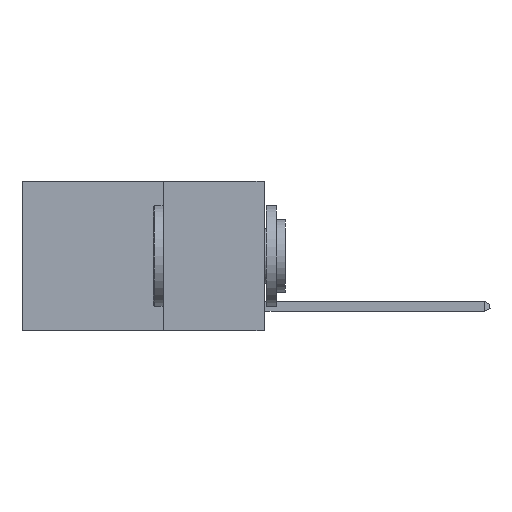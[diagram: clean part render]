
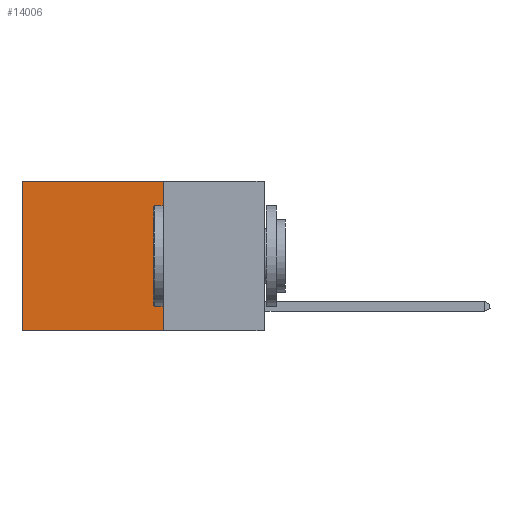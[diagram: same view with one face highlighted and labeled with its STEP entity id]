
A CAD part, left-side view. The second image highlights one B-rep face of the part: STEP entity #14006.
In plain terms, the highlighted planar face has unit normal (-1, 0, 0).
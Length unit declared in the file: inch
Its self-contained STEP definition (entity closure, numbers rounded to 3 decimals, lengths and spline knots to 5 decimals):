
#218 = DIRECTION ( 'NONE',  ( 0., 1., 0. ) ) ;
#774 = EDGE_CURVE ( 'NONE', #12785, #7428, #1896, .T. ) ;
#1178 = CARTESIAN_POINT ( 'NONE',  ( 0.2625, 0.25, 0. ) ) ;
#1499 = ORIENTED_EDGE ( 'NONE', *, *, #6304, .T. ) ;
#1896 = LINE ( 'NONE', #18213, #20270 ) ;
#2748 = EDGE_CURVE ( 'NONE', #5955, #7428, #11706, .T. ) ;
#3191 = PLANE ( 'NONE',  #17460 ) ;
#4919 = DIRECTION ( 'NONE',  ( 1., 0., 0. ) ) ;
#5217 = CARTESIAN_POINT ( 'NONE',  ( 0.2625, 0.6, 0. ) ) ;
#5929 = DIRECTION ( 'NONE',  ( 0., 0., -1. ) ) ;
#5955 = VERTEX_POINT ( 'NONE', #5217 ) ;
#6304 = EDGE_CURVE ( 'NONE', #12849, #5955, #6588, .T. ) ;
#6588 = LINE ( 'NONE', #6692, #6693 ) ;
#6692 = CARTESIAN_POINT ( 'NONE',  ( 0.2625, 0.25, 0. ) ) ;
#6693 = VECTOR ( 'NONE', #218, 39.37008 ) ;
#7428 = VERTEX_POINT ( 'NONE', #13947 ) ;
#7990 = ORIENTED_EDGE ( 'NONE', *, *, #17833, .F. ) ;
#8129 = DIRECTION ( 'NONE',  ( 0., 0., -1. ) ) ;
#10306 = CARTESIAN_POINT ( 'NONE',  ( 0.2625, 0.25, 0. ) ) ;
#11030 = EDGE_LOOP ( 'NONE', ( #17191, #18060, #7990, #1499 ) ) ;
#11706 = LINE ( 'NONE', #18285, #13507 ) ;
#12785 = VERTEX_POINT ( 'NONE', #21215 ) ;
#12849 = VERTEX_POINT ( 'NONE', #10306 ) ;
#13134 = FACE_OUTER_BOUND ( 'NONE', #11030, .T. ) ;
#13507 = VECTOR ( 'NONE', #8129, 39.37008 ) ;
#13947 = CARTESIAN_POINT ( 'NONE',  ( 0.2625, 0.6, -0.37 ) ) ;
#14006 = ADVANCED_FACE ( 'NONE', ( #13134 ), #3191, .F. ) ;
#14972 = CARTESIAN_POINT ( 'NONE',  ( 0.2625, 0.25, 0. ) ) ;
#17191 = ORIENTED_EDGE ( 'NONE', *, *, #2748, .T. ) ;
#17460 = AXIS2_PLACEMENT_3D ( 'NONE', #14972, #4919, #19929 ) ;
#17833 = EDGE_CURVE ( 'NONE', #12849, #12785, #20726, .T. ) ;
#18060 = ORIENTED_EDGE ( 'NONE', *, *, #774, .F. ) ;
#18213 = CARTESIAN_POINT ( 'NONE',  ( 0.2625, 0.25, -0.37 ) ) ;
#18285 = CARTESIAN_POINT ( 'NONE',  ( 0.2625, 0.6, 0. ) ) ;
#18408 = DIRECTION ( 'NONE',  ( 0., 1., 0. ) ) ;
#19929 = DIRECTION ( 'NONE',  ( 0., 0., -1. ) ) ;
#20110 = VECTOR ( 'NONE', #5929, 39.37008 ) ;
#20270 = VECTOR ( 'NONE', #18408, 39.37008 ) ;
#20726 = LINE ( 'NONE', #1178, #20110 ) ;
#21215 = CARTESIAN_POINT ( 'NONE',  ( 0.2625, 0.25, -0.37 ) ) ;
